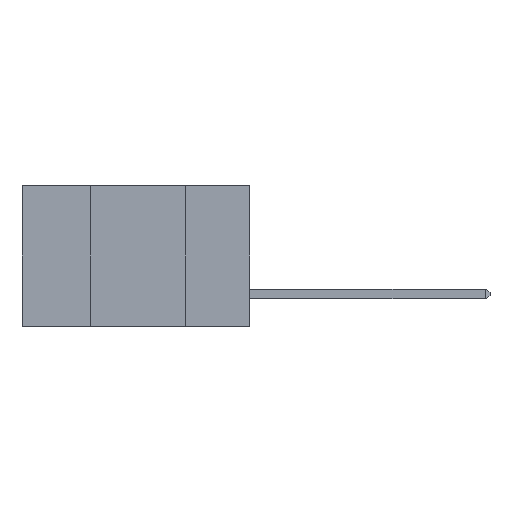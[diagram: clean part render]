
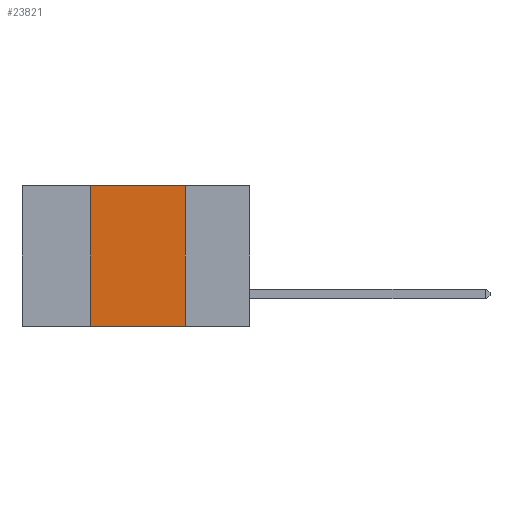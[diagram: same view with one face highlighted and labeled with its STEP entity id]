
A CAD part, left-side view. The second image highlights one B-rep face of the part: STEP entity #23821.
In plain terms, the highlighted planar face has unit normal (-1, 0, 0).
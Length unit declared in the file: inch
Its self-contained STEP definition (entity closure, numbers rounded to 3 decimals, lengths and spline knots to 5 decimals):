
#286 = VECTOR ( 'NONE', #6333, 39.37008 ) ;
#624 = VERTEX_POINT ( 'NONE', #22044 ) ;
#1204 = LINE ( 'NONE', #17688, #10887 ) ;
#1488 = DIRECTION ( 'NONE',  ( 0., 0., -1. ) ) ;
#2666 = LINE ( 'NONE', #22621, #22577 ) ;
#2717 = EDGE_CURVE ( 'NONE', #15137, #17774, #15142, .T. ) ;
#3055 = EDGE_CURVE ( 'NONE', #8648, #624, #2666, .T. ) ;
#3936 = PLANE ( 'NONE',  #14868 ) ;
#4340 = CARTESIAN_POINT ( 'NONE',  ( 0., 0.42, 0. ) ) ;
#4410 = EDGE_LOOP ( 'NONE', ( #19149, #18029, #23378, #16911 ) ) ;
#4687 = FACE_OUTER_BOUND ( 'NONE', #4410, .T. ) ;
#6333 = DIRECTION ( 'NONE',  ( 0., 0., 1. ) ) ;
#7880 = CARTESIAN_POINT ( 'NONE',  ( 0., 0.6, 0. ) ) ;
#8648 = VERTEX_POINT ( 'NONE', #21606 ) ;
#9503 = CARTESIAN_POINT ( 'NONE',  ( 0., 0.42, -0.37 ) ) ;
#9835 = DIRECTION ( 'NONE',  ( 0., 0., -1. ) ) ;
#10887 = VECTOR ( 'NONE', #19620, 39.37008 ) ;
#13538 = LINE ( 'NONE', #19431, #23104 ) ;
#14868 = AXIS2_PLACEMENT_3D ( 'NONE', #7880, #21323, #9835 ) ;
#15137 = VERTEX_POINT ( 'NONE', #9503 ) ;
#15142 = LINE ( 'NONE', #4340, #286 ) ;
#16911 = ORIENTED_EDGE ( 'NONE', *, *, #19896, .T. ) ;
#17688 = CARTESIAN_POINT ( 'NONE',  ( 0., 0.6, -0.37 ) ) ;
#17774 = VERTEX_POINT ( 'NONE', #22195 ) ;
#18029 = ORIENTED_EDGE ( 'NONE', *, *, #23241, .F. ) ;
#19149 = ORIENTED_EDGE ( 'NONE', *, *, #3055, .F. ) ;
#19431 = CARTESIAN_POINT ( 'NONE',  ( 0., 0.6, 0. ) ) ;
#19620 = DIRECTION ( 'NONE',  ( 0., -1., 0. ) ) ;
#19896 = EDGE_CURVE ( 'NONE', #15137, #624, #1204, .T. ) ;
#21323 = DIRECTION ( 'NONE',  ( 1., 0., 0. ) ) ;
#21340 = DIRECTION ( 'NONE',  ( 0., -1., 0. ) ) ;
#21606 = CARTESIAN_POINT ( 'NONE',  ( 0., 0.17, 0. ) ) ;
#22044 = CARTESIAN_POINT ( 'NONE',  ( 0., 0.17, -0.37 ) ) ;
#22195 = CARTESIAN_POINT ( 'NONE',  ( 0., 0.42, 0. ) ) ;
#22577 = VECTOR ( 'NONE', #1488, 39.37008 ) ;
#22621 = CARTESIAN_POINT ( 'NONE',  ( 0., 0.17, 0. ) ) ;
#23104 = VECTOR ( 'NONE', #21340, 39.37008 ) ;
#23241 = EDGE_CURVE ( 'NONE', #17774, #8648, #13538, .T. ) ;
#23378 = ORIENTED_EDGE ( 'NONE', *, *, #2717, .F. ) ;
#23821 = ADVANCED_FACE ( 'NONE', ( #4687 ), #3936, .F. ) ;
